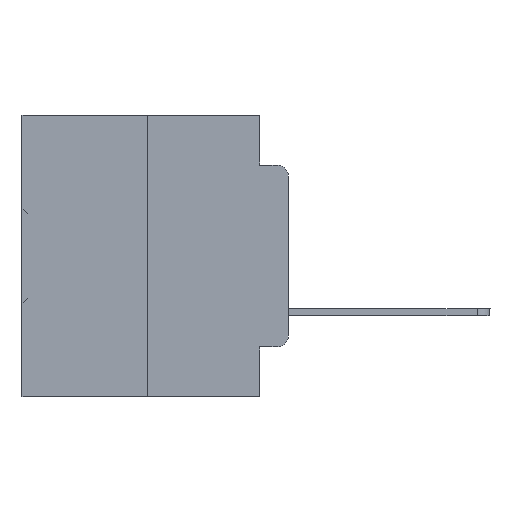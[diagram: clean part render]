
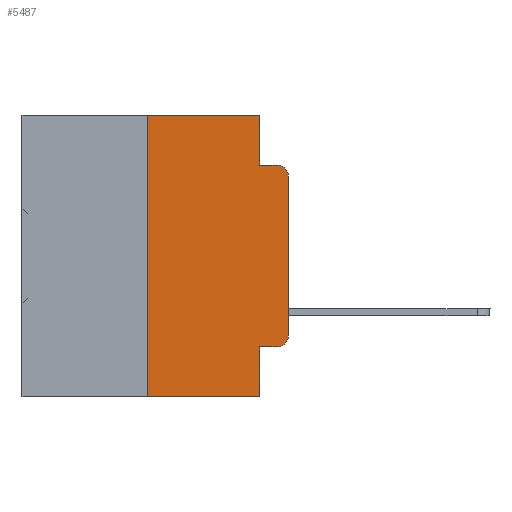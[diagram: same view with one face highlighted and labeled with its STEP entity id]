
A CAD part, left-side view. The second image highlights one B-rep face of the part: STEP entity #5487.
In plain terms, the highlighted planar face has unit normal (-1, 0, 0).
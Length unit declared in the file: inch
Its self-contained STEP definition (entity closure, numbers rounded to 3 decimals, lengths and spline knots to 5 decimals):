
#459 = LINE ( 'NONE', #6155, #4029 ) ;
#584 = LINE ( 'NONE', #11657, #35071 ) ;
#699 = CARTESIAN_POINT ( 'NONE',  ( 0., 0.473, -0.5 ) ) ;
#929 = DIRECTION ( 'NONE',  ( 0., 0., -1. ) ) ;
#989 = VECTOR ( 'NONE', #1018, 39.37008 ) ;
#1018 = DIRECTION ( 'NONE',  ( 0., 0., -1. ) ) ;
#1389 = ORIENTED_EDGE ( 'NONE', *, *, #13504, .F. ) ;
#1789 = VECTOR ( 'NONE', #17397, 39.37008 ) ;
#2285 = ORIENTED_EDGE ( 'NONE', *, *, #3010, .F. ) ;
#3010 = EDGE_CURVE ( 'NONE', #35047, #25719, #584, .T. ) ;
#3282 = DIRECTION ( 'NONE',  ( 0., 0., 1. ) ) ;
#3456 = CARTESIAN_POINT ( 'NONE',  ( 0., 0.25, 0. ) ) ;
#4019 = VERTEX_POINT ( 'NONE', #23862 ) ;
#4029 = VECTOR ( 'NONE', #31392, 39.37008 ) ;
#4498 = EDGE_CURVE ( 'NONE', #11726, #30498, #26085, .T. ) ;
#5356 = VERTEX_POINT ( 'NONE', #31153 ) ;
#5487 = ADVANCED_FACE ( 'NONE', ( #14589 ), #26367, .F. ) ;
#6155 = CARTESIAN_POINT ( 'NONE',  ( 0., 0.051, 0. ) ) ;
#6262 = CARTESIAN_POINT ( 'NONE',  ( 0., 0., 0. ) ) ;
#6362 = CARTESIAN_POINT ( 'NONE',  ( 0., 0.02, -0.0885 ) ) ;
#6452 = DIRECTION ( 'NONE',  ( 0., 0., 1. ) ) ;
#8098 = EDGE_CURVE ( 'NONE', #15874, #19671, #14575, .T. ) ;
#8565 = LINE ( 'NONE', #19809, #1789 ) ;
#9224 = ORIENTED_EDGE ( 'NONE', *, *, #35483, .F. ) ;
#10497 = DIRECTION ( 'NONE',  ( -1., 0., 0. ) ) ;
#11494 = CIRCLE ( 'NONE', #12655, 0.02 ) ;
#11657 = CARTESIAN_POINT ( 'NONE',  ( 0., 0.051, -0.0885 ) ) ;
#11726 = VERTEX_POINT ( 'NONE', #22108 ) ;
#11802 = CARTESIAN_POINT ( 'NONE',  ( 0., 0.051, -0.0885 ) ) ;
#12655 = AXIS2_PLACEMENT_3D ( 'NONE', #21916, #10497, #22288 ) ;
#13504 = EDGE_CURVE ( 'NONE', #5356, #35047, #459, .T. ) ;
#13743 = VERTEX_POINT ( 'NONE', #19416 ) ;
#14575 = LINE ( 'NONE', #6262, #20217 ) ;
#14589 = FACE_OUTER_BOUND ( 'NONE', #25875, .T. ) ;
#14670 = ORIENTED_EDGE ( 'NONE', *, *, #8098, .T. ) ;
#14825 = DIRECTION ( 'NONE',  ( 0., -1., 0. ) ) ;
#14940 = CARTESIAN_POINT ( 'NONE',  ( 0., 0.02, -0.1085 ) ) ;
#15142 = CARTESIAN_POINT ( 'NONE',  ( 0., 0.051, -0.5 ) ) ;
#15565 = CARTESIAN_POINT ( 'NONE',  ( 0., 0.051, -0.4115 ) ) ;
#15874 = VERTEX_POINT ( 'NONE', #29996 ) ;
#16806 = EDGE_CURVE ( 'NONE', #13743, #5356, #8565, .T. ) ;
#16891 = EDGE_CURVE ( 'NONE', #11726, #4019, #34874, .T. ) ;
#17208 = CIRCLE ( 'NONE', #18984, 0.02 ) ;
#17397 = DIRECTION ( 'NONE',  ( 0., -1., 0. ) ) ;
#17883 = DIRECTION ( 'NONE',  ( 1., 0., 0. ) ) ;
#18796 = ORIENTED_EDGE ( 'NONE', *, *, #28570, .T. ) ;
#18984 = AXIS2_PLACEMENT_3D ( 'NONE', #14940, #26178, #929 ) ;
#19416 = CARTESIAN_POINT ( 'NONE',  ( 0., 0.25, 0. ) ) ;
#19671 = VERTEX_POINT ( 'NONE', #19793 ) ;
#19759 = DIRECTION ( 'NONE',  ( 0., -1., 0. ) ) ;
#19793 = CARTESIAN_POINT ( 'NONE',  ( 0., 0., -0.1085 ) ) ;
#19809 = CARTESIAN_POINT ( 'NONE',  ( 0., 0.473, 0. ) ) ;
#20217 = VECTOR ( 'NONE', #6452, 39.37008 ) ;
#20281 = DIRECTION ( 'NONE',  ( 0., 0., -1. ) ) ;
#20785 = LINE ( 'NONE', #699, #30177 ) ;
#21826 = VECTOR ( 'NONE', #14825, 39.37008 ) ;
#21867 = ORIENTED_EDGE ( 'NONE', *, *, #25208, .T. ) ;
#21916 = CARTESIAN_POINT ( 'NONE',  ( 0., 0.02, -0.3915 ) ) ;
#22108 = CARTESIAN_POINT ( 'NONE',  ( 0., 0.051, -0.4115 ) ) ;
#22288 = DIRECTION ( 'NONE',  ( 0., 0., -1. ) ) ;
#23214 = ORIENTED_EDGE ( 'NONE', *, *, #4498, .F. ) ;
#23862 = CARTESIAN_POINT ( 'NONE',  ( 0., 0.02, -0.4115 ) ) ;
#24921 = EDGE_CURVE ( 'NONE', #19671, #25719, #17208, .T. ) ;
#25208 = EDGE_CURVE ( 'NONE', #25951, #30498, #20785, .T. ) ;
#25719 = VERTEX_POINT ( 'NONE', #6362 ) ;
#25875 = EDGE_LOOP ( 'NONE', ( #14670, #27963, #2285, #1389, #35107, #9224, #21867, #23214, #32662, #18796 ) ) ;
#25951 = VERTEX_POINT ( 'NONE', #28400 ) ;
#26085 = LINE ( 'NONE', #29211, #989 ) ;
#26178 = DIRECTION ( 'NONE',  ( -1., 0., 0. ) ) ;
#26367 = PLANE ( 'NONE',  #30231 ) ;
#27963 = ORIENTED_EDGE ( 'NONE', *, *, #24921, .T. ) ;
#28400 = CARTESIAN_POINT ( 'NONE',  ( 0., 0.25, -0.5 ) ) ;
#28516 = LINE ( 'NONE', #3456, #35948 ) ;
#28570 = EDGE_CURVE ( 'NONE', #4019, #15874, #11494, .T. ) ;
#29211 = CARTESIAN_POINT ( 'NONE',  ( 0., 0.051, 0. ) ) ;
#29996 = CARTESIAN_POINT ( 'NONE',  ( 0., 0., -0.3915 ) ) ;
#30177 = VECTOR ( 'NONE', #31823, 39.37008 ) ;
#30231 = AXIS2_PLACEMENT_3D ( 'NONE', #31869, #17883, #20281 ) ;
#30498 = VERTEX_POINT ( 'NONE', #15142 ) ;
#31153 = CARTESIAN_POINT ( 'NONE',  ( 0., 0.051, 0. ) ) ;
#31392 = DIRECTION ( 'NONE',  ( 0., 0., -1. ) ) ;
#31823 = DIRECTION ( 'NONE',  ( 0., -1., 0. ) ) ;
#31869 = CARTESIAN_POINT ( 'NONE',  ( 0., 0.473, 0. ) ) ;
#32662 = ORIENTED_EDGE ( 'NONE', *, *, #16891, .T. ) ;
#34874 = LINE ( 'NONE', #15565, #21826 ) ;
#35047 = VERTEX_POINT ( 'NONE', #11802 ) ;
#35071 = VECTOR ( 'NONE', #19759, 39.37008 ) ;
#35107 = ORIENTED_EDGE ( 'NONE', *, *, #16806, .F. ) ;
#35483 = EDGE_CURVE ( 'NONE', #25951, #13743, #28516, .T. ) ;
#35948 = VECTOR ( 'NONE', #3282, 39.37008 ) ;
